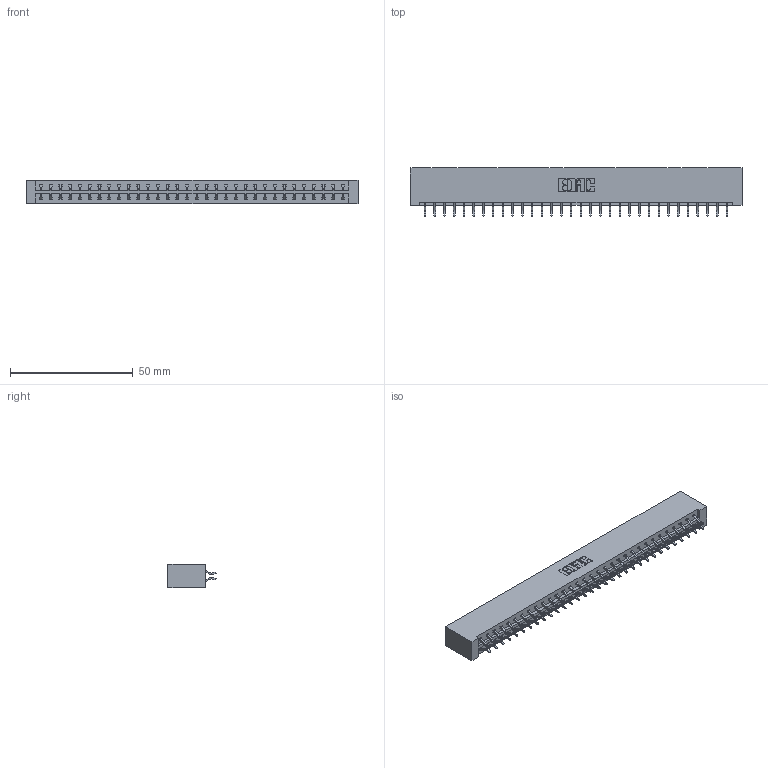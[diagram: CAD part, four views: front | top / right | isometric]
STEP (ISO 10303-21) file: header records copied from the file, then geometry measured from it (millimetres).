
FILE_DESCRIPTION (( 'STEP AP203' ), '1' );
FILE_NAME ('833-064-556-201.STEP', '2020-06-05T07:44:19', ( '' ), ( '' ), 'SwSTEP 2.0', 'SolidWorks 2020', '' );
FILE_SCHEMA (( 'CONFIG_CONTROL_DESIGN' ));
Length unit declared in the file: inch
Products named in the file (3): 833-064-556-201; 833 Part_Lugless; 345-292-001_556 Tail
Assembly tree (65 placements, depth 2):
  833-064-556-201
    833 Part_Lugless
    345-292-001_556 Tail  x64
Bounding box: 135.05 x 19.57 x 9.4 mm (x, y, z)
Volume: 14324.2 mm3; surface area: 16788.5 mm2
Topology: 65 solids, 65 shells, 3818 faces, 11359 edges, 7486 vertices
Faces by surface type: plane 2626, cylinder 1192
Entity records: 21823 total; most frequent: CARTESIAN_POINT 3642, ORIENTED_EDGE 3566, DIRECTION 3111, EDGE_CURVE 1783, LINE 1655, VECTOR 1655, VERTEX_POINT 1186, AXIS2_PLACEMENT_3D 728
